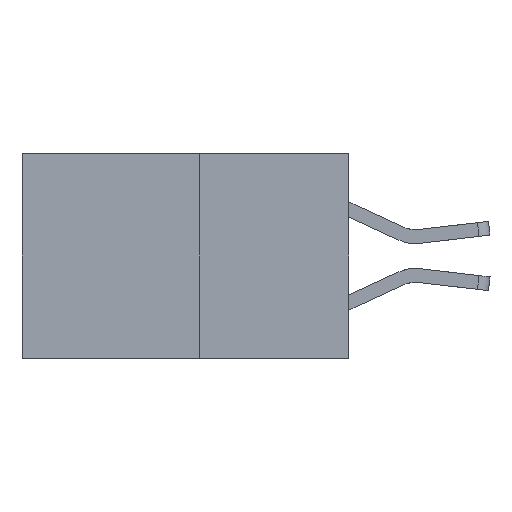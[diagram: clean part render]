
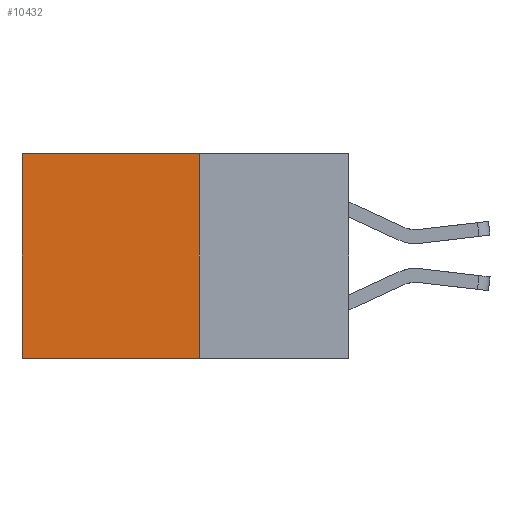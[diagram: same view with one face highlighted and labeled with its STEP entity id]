
A CAD part, left-side view. The second image highlights one B-rep face of the part: STEP entity #10432.
In plain terms, the highlighted planar face has unit normal (-1, 0, 0).
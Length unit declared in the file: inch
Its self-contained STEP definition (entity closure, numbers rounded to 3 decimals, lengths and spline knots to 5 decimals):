
#655 = VECTOR ( 'NONE', #4883, 39.37008 ) ;
#850 = DIRECTION ( 'NONE',  ( 1., 0., 0. ) ) ;
#892 = EDGE_CURVE ( 'NONE', #7847, #3838, #8050, .T. ) ;
#1794 = CARTESIAN_POINT ( 'NONE',  ( 0.277, 0.27, -0.37 ) ) ;
#2564 = VECTOR ( 'NONE', #11516, 39.37008 ) ;
#2815 = EDGE_CURVE ( 'NONE', #9057, #3838, #7750, .T. ) ;
#2909 = CARTESIAN_POINT ( 'NONE',  ( 0.277, 0.27, -0.37 ) ) ;
#3250 = EDGE_CURVE ( 'NONE', #11184, #7847, #5381, .T. ) ;
#3330 = LINE ( 'NONE', #2909, #10275 ) ;
#3696 = FACE_OUTER_BOUND ( 'NONE', #8338, .T. ) ;
#3792 = CARTESIAN_POINT ( 'NONE',  ( 0.277, 0.59, -0.37 ) ) ;
#3838 = VERTEX_POINT ( 'NONE', #3792 ) ;
#3860 = DIRECTION ( 'NONE',  ( 0., 0., -1. ) ) ;
#4883 = DIRECTION ( 'NONE',  ( 0., 0., -1. ) ) ;
#5381 = LINE ( 'NONE', #11441, #2564 ) ;
#5390 = VECTOR ( 'NONE', #8697, 39.37008 ) ;
#6144 = AXIS2_PLACEMENT_3D ( 'NONE', #1794, #850, #7355 ) ;
#6461 = CARTESIAN_POINT ( 'NONE',  ( 0.277, 0.59, 0. ) ) ;
#6824 = CARTESIAN_POINT ( 'NONE',  ( 0.277, 0.59, -0.37 ) ) ;
#7355 = DIRECTION ( 'NONE',  ( 0., 0., -1. ) ) ;
#7422 = CARTESIAN_POINT ( 'NONE',  ( 0.277, 0.27, -0.37 ) ) ;
#7750 = LINE ( 'NONE', #7422, #5390 ) ;
#7847 = VERTEX_POINT ( 'NONE', #6461 ) ;
#8050 = LINE ( 'NONE', #6824, #655 ) ;
#8338 = EDGE_LOOP ( 'NONE', ( #9190, #9034, #9014, #8952 ) ) ;
#8697 = DIRECTION ( 'NONE',  ( 0., 1., 0. ) ) ;
#8952 = ORIENTED_EDGE ( 'NONE', *, *, #3250, .T. ) ;
#9014 = ORIENTED_EDGE ( 'NONE', *, *, #9038, .F. ) ;
#9034 = ORIENTED_EDGE ( 'NONE', *, *, #2815, .F. ) ;
#9038 = EDGE_CURVE ( 'NONE', #11184, #9057, #3330, .T. ) ;
#9057 = VERTEX_POINT ( 'NONE', #11028 ) ;
#9190 = ORIENTED_EDGE ( 'NONE', *, *, #892, .T. ) ;
#10275 = VECTOR ( 'NONE', #3860, 39.37008 ) ;
#10432 = ADVANCED_FACE ( 'NONE', ( #3696 ), #10851, .F. ) ;
#10851 = PLANE ( 'NONE',  #6144 ) ;
#11028 = CARTESIAN_POINT ( 'NONE',  ( 0.277, 0.27, -0.37 ) ) ;
#11184 = VERTEX_POINT ( 'NONE', #11693 ) ;
#11441 = CARTESIAN_POINT ( 'NONE',  ( 0.277, 0.27, 0. ) ) ;
#11516 = DIRECTION ( 'NONE',  ( 0., 1., 0. ) ) ;
#11693 = CARTESIAN_POINT ( 'NONE',  ( 0.277, 0.27, 0. ) ) ;
